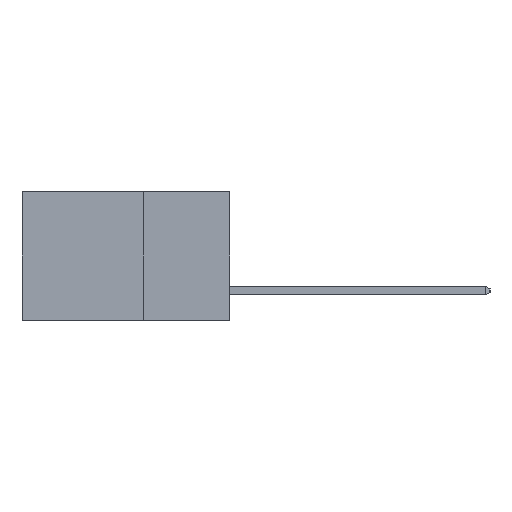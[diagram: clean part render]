
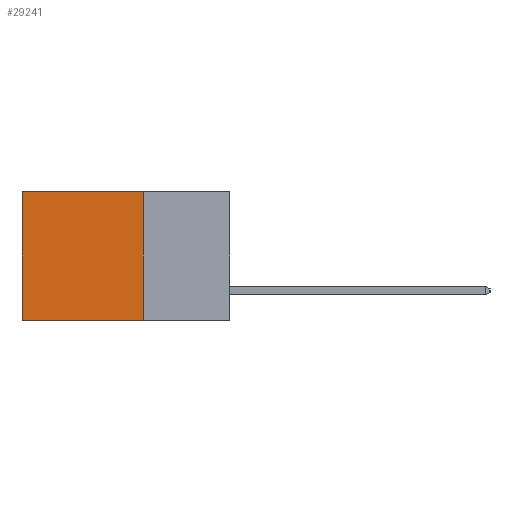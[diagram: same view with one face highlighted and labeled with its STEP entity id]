
A CAD part, left-side view. The second image highlights one B-rep face of the part: STEP entity #29241.
In plain terms, the highlighted planar face has unit normal (-1, 0, 0).
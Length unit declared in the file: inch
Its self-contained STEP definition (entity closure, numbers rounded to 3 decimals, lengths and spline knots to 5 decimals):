
#450 = EDGE_LOOP ( 'NONE', ( #30407, #17450, #28050, #16553 ) ) ;
#588 = CARTESIAN_POINT ( 'NONE',  ( 0.298, 0.25, 0. ) ) ;
#1965 = VERTEX_POINT ( 'NONE', #1999 ) ;
#1999 = CARTESIAN_POINT ( 'NONE',  ( 0.298, 0.25, -0.37 ) ) ;
#2529 = LINE ( 'NONE', #11629, #15754 ) ;
#2542 = CARTESIAN_POINT ( 'NONE',  ( 0.298, 0.6, -0.37 ) ) ;
#2918 = CARTESIAN_POINT ( 'NONE',  ( 0.298, 0.25, -0.37 ) ) ;
#4393 = CARTESIAN_POINT ( 'NONE',  ( 0.298, 0.25, 0. ) ) ;
#5193 = AXIS2_PLACEMENT_3D ( 'NONE', #5825, #23051, #8321 ) ;
#5825 = CARTESIAN_POINT ( 'NONE',  ( 0.298, 0.25, 0. ) ) ;
#7720 = LINE ( 'NONE', #2918, #26581 ) ;
#8321 = DIRECTION ( 'NONE',  ( 0., 0., -1. ) ) ;
#10434 = DIRECTION ( 'NONE',  ( 0., 1., 0. ) ) ;
#11355 = EDGE_CURVE ( 'NONE', #13801, #24289, #19775, .T. ) ;
#11629 = CARTESIAN_POINT ( 'NONE',  ( 0.298, 0.25, 0. ) ) ;
#11639 = CARTESIAN_POINT ( 'NONE',  ( 0.298, 0.6, 0. ) ) ;
#13801 = VERTEX_POINT ( 'NONE', #16484 ) ;
#15490 = DIRECTION ( 'NONE',  ( 0., 0., -1. ) ) ;
#15754 = VECTOR ( 'NONE', #28633, 39.37008 ) ;
#16140 = FACE_OUTER_BOUND ( 'NONE', #450, .T. ) ;
#16484 = CARTESIAN_POINT ( 'NONE',  ( 0.298, 0.6, 0. ) ) ;
#16553 = ORIENTED_EDGE ( 'NONE', *, *, #17511, .T. ) ;
#16612 = DIRECTION ( 'NONE',  ( 0., 0., -1. ) ) ;
#17450 = ORIENTED_EDGE ( 'NONE', *, *, #20452, .F. ) ;
#17511 = EDGE_CURVE ( 'NONE', #22614, #13801, #2529, .T. ) ;
#18194 = PLANE ( 'NONE',  #5193 ) ;
#19775 = LINE ( 'NONE', #11639, #26262 ) ;
#20452 = EDGE_CURVE ( 'NONE', #1965, #24289, #7720, .T. ) ;
#22614 = VERTEX_POINT ( 'NONE', #4393 ) ;
#22900 = EDGE_CURVE ( 'NONE', #22614, #1965, #24088, .T. ) ;
#23051 = DIRECTION ( 'NONE',  ( 1., 0., 0. ) ) ;
#24088 = LINE ( 'NONE', #588, #29018 ) ;
#24289 = VERTEX_POINT ( 'NONE', #2542 ) ;
#26262 = VECTOR ( 'NONE', #16612, 39.37008 ) ;
#26581 = VECTOR ( 'NONE', #10434, 39.37008 ) ;
#28050 = ORIENTED_EDGE ( 'NONE', *, *, #22900, .F. ) ;
#28633 = DIRECTION ( 'NONE',  ( 0., 1., 0. ) ) ;
#29018 = VECTOR ( 'NONE', #15490, 39.37008 ) ;
#29241 = ADVANCED_FACE ( 'NONE', ( #16140 ), #18194, .F. ) ;
#30407 = ORIENTED_EDGE ( 'NONE', *, *, #11355, .T. ) ;
